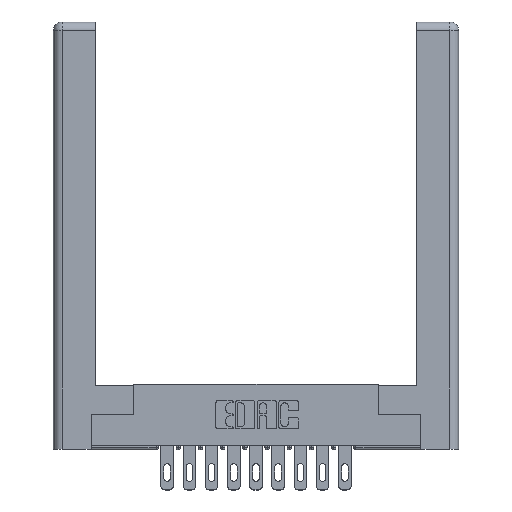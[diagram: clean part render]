
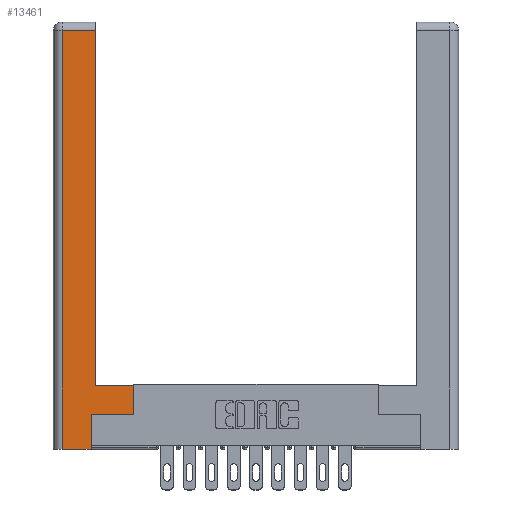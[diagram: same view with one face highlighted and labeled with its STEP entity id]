
A CAD part, top view. The second image highlights one B-rep face of the part: STEP entity #13461.
In plain terms, the highlighted planar face has unit normal (0, 0, 1).
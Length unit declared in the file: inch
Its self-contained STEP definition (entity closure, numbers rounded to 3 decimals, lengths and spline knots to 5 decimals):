
#37 = CARTESIAN_POINT ( 'NONE',  ( 0.565, 0.45, 0. ) ) ;
#299 = DIRECTION ( 'NONE',  ( 0., 1., 0. ) ) ;
#629 = CARTESIAN_POINT ( 'NONE',  ( 0.295, 2.94, 0. ) ) ;
#724 = ORIENTED_EDGE ( 'NONE', *, *, #969, .T. ) ;
#964 = LINE ( 'NONE', #3587, #11278 ) ;
#969 = EDGE_CURVE ( 'NONE', #6142, #13813, #10711, .T. ) ;
#1376 = DIRECTION ( 'NONE',  ( 1., 0., 0. ) ) ;
#1579 = LINE ( 'NONE', #8595, #14292 ) ;
#1584 = CARTESIAN_POINT ( 'NONE',  ( 0.295, 0.45, 0. ) ) ;
#1832 = VECTOR ( 'NONE', #14786, 39.37008 ) ;
#2363 = CARTESIAN_POINT ( 'NONE',  ( 0.0615, 2.94, 0. ) ) ;
#2485 = CARTESIAN_POINT ( 'NONE',  ( 0., 0., 0. ) ) ;
#2536 = CARTESIAN_POINT ( 'NONE',  ( 0.565, 0.245, 0. ) ) ;
#3011 = ORIENTED_EDGE ( 'NONE', *, *, #9169, .T. ) ;
#3120 = VECTOR ( 'NONE', #14553, 39.37008 ) ;
#3169 = AXIS2_PLACEMENT_3D ( 'NONE', #2485, #3742, #10170 ) ;
#3199 = CARTESIAN_POINT ( 'NONE',  ( 0.265, 0.245, 0. ) ) ;
#3256 = CARTESIAN_POINT ( 'NONE',  ( 0.295, 0.45, 0. ) ) ;
#3433 = VERTEX_POINT ( 'NONE', #12436 ) ;
#3587 = CARTESIAN_POINT ( 'NONE',  ( 0.265, 0., 0. ) ) ;
#3742 = DIRECTION ( 'NONE',  ( 0., 0., -1. ) ) ;
#3994 = CARTESIAN_POINT ( 'NONE',  ( 0.0615, 0., 0. ) ) ;
#4929 = ORIENTED_EDGE ( 'NONE', *, *, #16148, .T. ) ;
#5602 = DIRECTION ( 'NONE',  ( -1., 0., 0. ) ) ;
#5616 = VECTOR ( 'NONE', #5602, 39.37008 ) ;
#5894 = ORIENTED_EDGE ( 'NONE', *, *, #12480, .T. ) ;
#6142 = VERTEX_POINT ( 'NONE', #1584 ) ;
#6256 = CARTESIAN_POINT ( 'NONE',  ( 0.0615, 0., 0. ) ) ;
#6695 = VERTEX_POINT ( 'NONE', #10786 ) ;
#7041 = ORIENTED_EDGE ( 'NONE', *, *, #16076, .T. ) ;
#7388 = DIRECTION ( 'NONE',  ( 1., 0., 0. ) ) ;
#7598 = DIRECTION ( 'NONE',  ( 0., -1., 0. ) ) ;
#7905 = EDGE_CURVE ( 'NONE', #13813, #10970, #12557, .T. ) ;
#8227 = CARTESIAN_POINT ( 'NONE',  ( 0.0615, 2.94, 0. ) ) ;
#8317 = EDGE_CURVE ( 'NONE', #12854, #3433, #10974, .T. ) ;
#8324 = LINE ( 'NONE', #6256, #10110 ) ;
#8595 = CARTESIAN_POINT ( 'NONE',  ( 0.265, 0.245, 0. ) ) ;
#9076 = VERTEX_POINT ( 'NONE', #3199 ) ;
#9169 = EDGE_CURVE ( 'NONE', #6695, #9076, #1579, .T. ) ;
#9488 = LINE ( 'NONE', #2536, #11835 ) ;
#9904 = CARTESIAN_POINT ( 'NONE',  ( 0.565, 0.245, 0. ) ) ;
#10110 = VECTOR ( 'NONE', #7598, 39.37008 ) ;
#10170 = DIRECTION ( 'NONE',  ( -1., 0., 0. ) ) ;
#10603 = ORIENTED_EDGE ( 'NONE', *, *, #7905, .T. ) ;
#10711 = LINE ( 'NONE', #14150, #16232 ) ;
#10786 = CARTESIAN_POINT ( 'NONE',  ( 0.265, 0., 0. ) ) ;
#10970 = VERTEX_POINT ( 'NONE', #2363 ) ;
#10974 = LINE ( 'NONE', #37, #1832 ) ;
#11278 = VECTOR ( 'NONE', #7388, 39.37008 ) ;
#11505 = ORIENTED_EDGE ( 'NONE', *, *, #8317, .T. ) ;
#11835 = VECTOR ( 'NONE', #1376, 39.37008 ) ;
#11850 = LINE ( 'NONE', #3256, #3120 ) ;
#12091 = EDGE_CURVE ( 'NONE', #3433, #6142, #11850, .T. ) ;
#12408 = DIRECTION ( 'NONE',  ( 0., 1., 0. ) ) ;
#12436 = CARTESIAN_POINT ( 'NONE',  ( 0.565, 0.45, 0. ) ) ;
#12480 = EDGE_CURVE ( 'NONE', #9076, #12854, #9488, .T. ) ;
#12549 = EDGE_LOOP ( 'NONE', ( #724, #10603, #4929, #7041, #3011, #5894, #11505, #14930 ) ) ;
#12557 = LINE ( 'NONE', #8227, #5616 ) ;
#12854 = VERTEX_POINT ( 'NONE', #9904 ) ;
#13461 = ADVANCED_FACE ( 'NONE', ( #14337 ), #14010, .F. ) ;
#13813 = VERTEX_POINT ( 'NONE', #629 ) ;
#14010 = PLANE ( 'NONE',  #3169 ) ;
#14150 = CARTESIAN_POINT ( 'NONE',  ( 0.295, 3., 0. ) ) ;
#14292 = VECTOR ( 'NONE', #12408, 39.37008 ) ;
#14337 = FACE_OUTER_BOUND ( 'NONE', #12549, .T. ) ;
#14553 = DIRECTION ( 'NONE',  ( -1., 0., 0. ) ) ;
#14786 = DIRECTION ( 'NONE',  ( 0., 1., 0. ) ) ;
#14930 = ORIENTED_EDGE ( 'NONE', *, *, #12091, .T. ) ;
#15899 = VERTEX_POINT ( 'NONE', #3994 ) ;
#16076 = EDGE_CURVE ( 'NONE', #15899, #6695, #964, .T. ) ;
#16148 = EDGE_CURVE ( 'NONE', #10970, #15899, #8324, .T. ) ;
#16232 = VECTOR ( 'NONE', #299, 39.37008 ) ;
